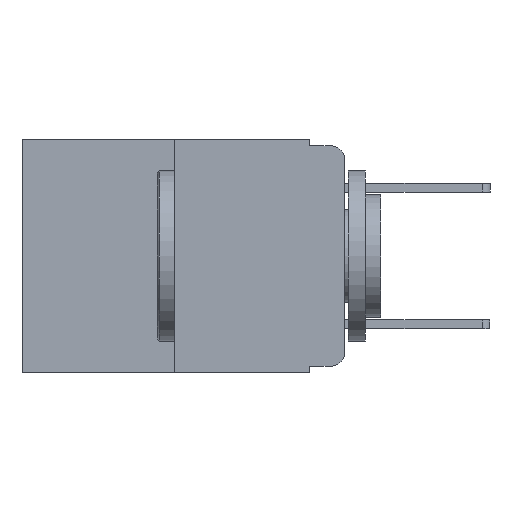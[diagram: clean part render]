
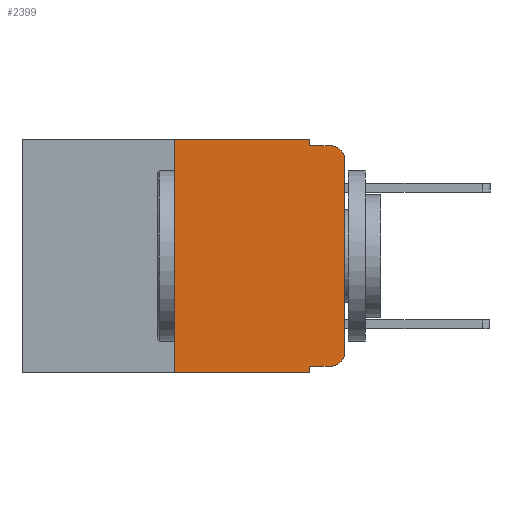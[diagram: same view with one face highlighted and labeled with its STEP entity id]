
A CAD part, left-side view. The second image highlights one B-rep face of the part: STEP entity #2399.
In plain terms, the highlighted planar face has unit normal (-1, 0, 0).
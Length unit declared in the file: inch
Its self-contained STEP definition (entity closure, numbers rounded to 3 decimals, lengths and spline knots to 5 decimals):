
#156 = LINE ( 'NONE', #12321, #9054 ) ;
#681 = CARTESIAN_POINT ( 'NONE',  ( 0., 0.473, -0.343 ) ) ;
#1530 = CARTESIAN_POINT ( 'NONE',  ( 0., 0.051, -0.343 ) ) ;
#2033 = CIRCLE ( 'NONE', #12769, 0.02 ) ;
#2399 = ADVANCED_FACE ( 'NONE', ( #3174 ), #6418, .F. ) ;
#2498 = EDGE_CURVE ( 'NONE', #5682, #13065, #15574, .T. ) ;
#2544 = VECTOR ( 'NONE', #14931, 39.37008 ) ;
#2892 = EDGE_CURVE ( 'NONE', #16597, #16698, #16873, .T. ) ;
#3174 = FACE_OUTER_BOUND ( 'NONE', #10185, .T. ) ;
#3223 = EDGE_CURVE ( 'NONE', #14847, #10457, #156, .T. ) ;
#3227 = EDGE_CURVE ( 'NONE', #10457, #9201, #4632, .T. ) ;
#3250 = EDGE_CURVE ( 'NONE', #14948, #9201, #11296, .T. ) ;
#3254 = EDGE_CURVE ( 'NONE', #13065, #14948, #3629, .T. ) ;
#3284 = EDGE_CURVE ( 'NONE', #16597, #5682, #6801, .T. ) ;
#3286 = EDGE_CURVE ( 'NONE', #18019, #16698, #14210, .T. ) ;
#3288 = EDGE_CURVE ( 'NONE', #18019, #13257, #17049, .T. ) ;
#3290 = EDGE_CURVE ( 'NONE', #13257, #14847, #2033, .T. ) ;
#3629 = LINE ( 'NONE', #9874, #10909 ) ;
#3856 = DIRECTION ( 'NONE',  ( 0., 0., 1. ) ) ;
#3873 = CARTESIAN_POINT ( 'NONE',  ( 0., 0.02, -0.333 ) ) ;
#4632 = CIRCLE ( 'NONE', #5393, 0.02 ) ;
#4654 = CARTESIAN_POINT ( 'NONE',  ( 0., 0.473, 0. ) ) ;
#5118 = ORIENTED_EDGE ( 'NONE', *, *, #3223, .T. ) ;
#5152 = ORIENTED_EDGE ( 'NONE', *, *, #3227, .T. ) ;
#5359 = ORIENTED_EDGE ( 'NONE', *, *, #3250, .F. ) ;
#5393 = AXIS2_PLACEMENT_3D ( 'NONE', #6981, #15997, #8458 ) ;
#5462 = ORIENTED_EDGE ( 'NONE', *, *, #3254, .F. ) ;
#5496 = CARTESIAN_POINT ( 'NONE',  ( 0., 0.051, -0.01 ) ) ;
#5635 = CARTESIAN_POINT ( 'NONE',  ( 0., 0.051, 0. ) ) ;
#5682 = VERTEX_POINT ( 'NONE', #17130 ) ;
#5701 = CARTESIAN_POINT ( 'NONE',  ( 0., 0.02, -0.313 ) ) ;
#5801 = ORIENTED_EDGE ( 'NONE', *, *, #2498, .F. ) ;
#5890 = ORIENTED_EDGE ( 'NONE', *, *, #3284, .F. ) ;
#6066 = ORIENTED_EDGE ( 'NONE', *, *, #2892, .T. ) ;
#6101 = ORIENTED_EDGE ( 'NONE', *, *, #3286, .F. ) ;
#6221 = ORIENTED_EDGE ( 'NONE', *, *, #3288, .T. ) ;
#6418 = PLANE ( 'NONE',  #9873 ) ;
#6437 = CARTESIAN_POINT ( 'NONE',  ( 0., 0.051, 0. ) ) ;
#6455 = ORIENTED_EDGE ( 'NONE', *, *, #3290, .T. ) ;
#6801 = LINE ( 'NONE', #8566, #2544 ) ;
#6981 = CARTESIAN_POINT ( 'NONE',  ( 0., 0.02, -0.03 ) ) ;
#7089 = DIRECTION ( 'NONE',  ( 0., 0., -1. ) ) ;
#7167 = DIRECTION ( 'NONE',  ( 0., 0., -1. ) ) ;
#7230 = DIRECTION ( 'NONE',  ( 0., 0., -1. ) ) ;
#7279 = DIRECTION ( 'NONE',  ( 0., -1., 0. ) ) ;
#7351 = CARTESIAN_POINT ( 'NONE',  ( 0., 0., -0.313 ) ) ;
#7542 = CARTESIAN_POINT ( 'NONE',  ( 0., 0.051, -0.01 ) ) ;
#7569 = VECTOR ( 'NONE', #7279, 39.37008 ) ;
#7586 = DIRECTION ( 'NONE',  ( 1., 0., 0. ) ) ;
#8458 = DIRECTION ( 'NONE',  ( 0., 0., -1. ) ) ;
#8512 = DIRECTION ( 'NONE',  ( 0., 0., -1. ) ) ;
#8566 = CARTESIAN_POINT ( 'NONE',  ( 0., 0.25, 0. ) ) ;
#8588 = CARTESIAN_POINT ( 'NONE',  ( 0., 0.051, -0.333 ) ) ;
#9054 = VECTOR ( 'NONE', #3856, 39.37008 ) ;
#9201 = VERTEX_POINT ( 'NONE', #15895 ) ;
#9240 = CARTESIAN_POINT ( 'NONE',  ( 0., 0.473, 0. ) ) ;
#9821 = DIRECTION ( 'NONE',  ( 0., -1., 0. ) ) ;
#9873 = AXIS2_PLACEMENT_3D ( 'NONE', #4654, #7586, #7089 ) ;
#9874 = CARTESIAN_POINT ( 'NONE',  ( 0., 0.051, 0. ) ) ;
#10103 = VECTOR ( 'NONE', #17371, 39.37008 ) ;
#10185 = EDGE_LOOP ( 'NONE', ( #5118, #5152, #5359, #5462, #5801, #5890, #6066, #6101, #6221, #6455 ) ) ;
#10457 = VERTEX_POINT ( 'NONE', #17905 ) ;
#10499 = VECTOR ( 'NONE', #7167, 39.37008 ) ;
#10728 = VECTOR ( 'NONE', #11229, 39.37008 ) ;
#10909 = VECTOR ( 'NONE', #8512, 39.37008 ) ;
#11215 = CARTESIAN_POINT ( 'NONE',  ( 0., 0.051, -0.333 ) ) ;
#11229 = DIRECTION ( 'NONE',  ( 0., -1., 0. ) ) ;
#11296 = LINE ( 'NONE', #5496, #14582 ) ;
#12321 = CARTESIAN_POINT ( 'NONE',  ( 0., 0., 0. ) ) ;
#12769 = AXIS2_PLACEMENT_3D ( 'NONE', #5701, #14979, #7230 ) ;
#13019 = CARTESIAN_POINT ( 'NONE',  ( 0., 0.25, -0.343 ) ) ;
#13065 = VERTEX_POINT ( 'NONE', #6437 ) ;
#13257 = VERTEX_POINT ( 'NONE', #3873 ) ;
#14210 = LINE ( 'NONE', #5635, #10499 ) ;
#14582 = VECTOR ( 'NONE', #9821, 39.37008 ) ;
#14847 = VERTEX_POINT ( 'NONE', #7351 ) ;
#14931 = DIRECTION ( 'NONE',  ( 0., 0., 1. ) ) ;
#14948 = VERTEX_POINT ( 'NONE', #7542 ) ;
#14979 = DIRECTION ( 'NONE',  ( -1., 0., 0. ) ) ;
#15574 = LINE ( 'NONE', #9240, #7569 ) ;
#15895 = CARTESIAN_POINT ( 'NONE',  ( 0., 0.02, -0.01 ) ) ;
#15997 = DIRECTION ( 'NONE',  ( -1., 0., 0. ) ) ;
#16597 = VERTEX_POINT ( 'NONE', #13019 ) ;
#16698 = VERTEX_POINT ( 'NONE', #1530 ) ;
#16873 = LINE ( 'NONE', #681, #10728 ) ;
#17049 = LINE ( 'NONE', #11215, #10103 ) ;
#17130 = CARTESIAN_POINT ( 'NONE',  ( 0., 0.25, 0. ) ) ;
#17371 = DIRECTION ( 'NONE',  ( 0., -1., 0. ) ) ;
#17905 = CARTESIAN_POINT ( 'NONE',  ( 0., 0., -0.03 ) ) ;
#18019 = VERTEX_POINT ( 'NONE', #8588 ) ;
